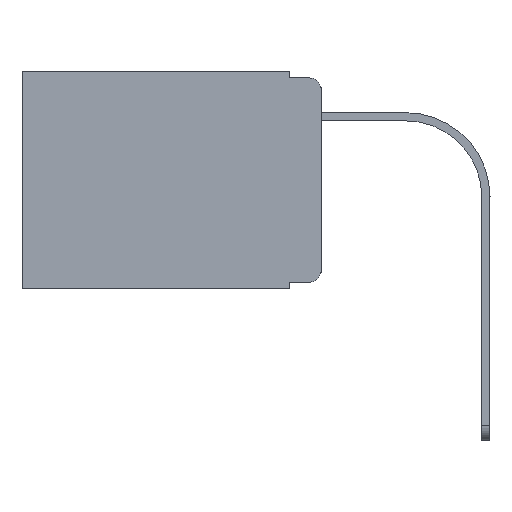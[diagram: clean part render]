
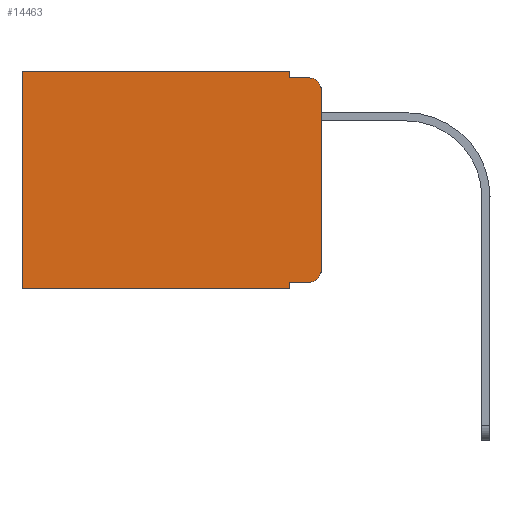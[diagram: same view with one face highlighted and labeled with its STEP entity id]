
A CAD part, left-side view. The second image highlights one B-rep face of the part: STEP entity #14463.
In plain terms, the highlighted planar face has unit normal (-1, 0, 0).
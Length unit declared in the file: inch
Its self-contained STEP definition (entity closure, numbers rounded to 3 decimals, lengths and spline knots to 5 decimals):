
#223 = CARTESIAN_POINT ( 'NONE',  ( 0.298, 0.051, -0.343 ) ) ;
#326 = EDGE_CURVE ( 'NONE', #18055, #405, #14141, .T. ) ;
#405 = VERTEX_POINT ( 'NONE', #223 ) ;
#505 = DIRECTION ( 'NONE',  ( 0., -1., 0. ) ) ;
#892 = DIRECTION ( 'NONE',  ( 0., 0., -1. ) ) ;
#959 = ORIENTED_EDGE ( 'NONE', *, *, #8449, .T. ) ;
#1194 = EDGE_CURVE ( 'NONE', #11760, #6548, #15734, .T. ) ;
#1338 = VERTEX_POINT ( 'NONE', #5907 ) ;
#1378 = DIRECTION ( 'NONE',  ( 0., 0., -1. ) ) ;
#1798 = FACE_OUTER_BOUND ( 'NONE', #3406, .T. ) ;
#2036 = VECTOR ( 'NONE', #18514, 39.37008 ) ;
#2287 = CARTESIAN_POINT ( 'NONE',  ( 0.298, 0., -0.343 ) ) ;
#2898 = DIRECTION ( 'NONE',  ( -1., 0., 0. ) ) ;
#3130 = DIRECTION ( 'NONE',  ( -1., 0., 0. ) ) ;
#3148 = VERTEX_POINT ( 'NONE', #5016 ) ;
#3279 = VECTOR ( 'NONE', #8430, 39.37008 ) ;
#3323 = CARTESIAN_POINT ( 'NONE',  ( 0.298, 0., 0. ) ) ;
#3406 = EDGE_LOOP ( 'NONE', ( #13383, #18698, #4146, #14200, #959, #3920, #7144, #18439, #6387, #9350 ) ) ;
#3530 = DIRECTION ( 'NONE',  ( 0., -1., 0. ) ) ;
#3554 = VECTOR ( 'NONE', #1378, 39.37008 ) ;
#3920 = ORIENTED_EDGE ( 'NONE', *, *, #1194, .T. ) ;
#3970 = VERTEX_POINT ( 'NONE', #10980 ) ;
#4146 = ORIENTED_EDGE ( 'NONE', *, *, #13550, .F. ) ;
#4601 = VECTOR ( 'NONE', #12641, 39.37008 ) ;
#4759 = VECTOR ( 'NONE', #505, 39.37008 ) ;
#4963 = LINE ( 'NONE', #7815, #9083 ) ;
#5016 = CARTESIAN_POINT ( 'NONE',  ( 0.298, 0., -0.03 ) ) ;
#5543 = LINE ( 'NONE', #2287, #2036 ) ;
#5906 = CARTESIAN_POINT ( 'NONE',  ( 0.298, 0.473, 0. ) ) ;
#5907 = CARTESIAN_POINT ( 'NONE',  ( 0.298, 0., -0.313 ) ) ;
#6193 = DIRECTION ( 'NONE',  ( 0., 0., -1. ) ) ;
#6314 = DIRECTION ( 'NONE',  ( 0., 1., 0. ) ) ;
#6387 = ORIENTED_EDGE ( 'NONE', *, *, #10122, .T. ) ;
#6539 = AXIS2_PLACEMENT_3D ( 'NONE', #17999, #3130, #7419 ) ;
#6548 = VERTEX_POINT ( 'NONE', #8036 ) ;
#6811 = CARTESIAN_POINT ( 'NONE',  ( 0.298, 0.051, 0. ) ) ;
#7144 = ORIENTED_EDGE ( 'NONE', *, *, #14064, .F. ) ;
#7419 = DIRECTION ( 'NONE',  ( 0., 0., -1. ) ) ;
#7556 = EDGE_CURVE ( 'NONE', #18207, #1338, #9958, .T. ) ;
#7567 = EDGE_CURVE ( 'NONE', #12636, #14679, #10074, .T. ) ;
#7608 = PLANE ( 'NONE',  #8438 ) ;
#7815 = CARTESIAN_POINT ( 'NONE',  ( 0.298, 0.051, -0.333 ) ) ;
#7850 = VECTOR ( 'NONE', #6314, 39.37008 ) ;
#7851 = LINE ( 'NONE', #11117, #18290 ) ;
#7915 = EDGE_CURVE ( 'NONE', #3148, #1338, #7851, .T. ) ;
#8036 = CARTESIAN_POINT ( 'NONE',  ( 0.298, 0.473, -0.343 ) ) ;
#8372 = CARTESIAN_POINT ( 'NONE',  ( 0.298, 0.051, -0.333 ) ) ;
#8430 = DIRECTION ( 'NONE',  ( 0., 0., -1. ) ) ;
#8438 = AXIS2_PLACEMENT_3D ( 'NONE', #3323, #18110, #6193 ) ;
#8449 = EDGE_CURVE ( 'NONE', #12636, #11760, #9181, .T. ) ;
#9083 = VECTOR ( 'NONE', #3530, 39.37008 ) ;
#9181 = LINE ( 'NONE', #17942, #7850 ) ;
#9350 = ORIENTED_EDGE ( 'NONE', *, *, #7556, .T. ) ;
#9958 = CIRCLE ( 'NONE', #18896, 0.02 ) ;
#10074 = LINE ( 'NONE', #18841, #3554 ) ;
#10122 = EDGE_CURVE ( 'NONE', #18055, #18207, #4963, .T. ) ;
#10980 = CARTESIAN_POINT ( 'NONE',  ( 0.298, 0.02, -0.01 ) ) ;
#11117 = CARTESIAN_POINT ( 'NONE',  ( 0.298, 0., 0. ) ) ;
#11236 = DIRECTION ( 'NONE',  ( 0., 0., -1. ) ) ;
#11442 = CARTESIAN_POINT ( 'NONE',  ( 0.298, 0.051, -0.01 ) ) ;
#11522 = CARTESIAN_POINT ( 'NONE',  ( 0.298, 0.02, -0.313 ) ) ;
#11734 = CARTESIAN_POINT ( 'NONE',  ( 0.298, 0.02, -0.333 ) ) ;
#11735 = CIRCLE ( 'NONE', #6539, 0.02 ) ;
#11760 = VERTEX_POINT ( 'NONE', #5906 ) ;
#11774 = EDGE_CURVE ( 'NONE', #3148, #3970, #11735, .T. ) ;
#12636 = VERTEX_POINT ( 'NONE', #16598 ) ;
#12641 = DIRECTION ( 'NONE',  ( 0., 0., -1. ) ) ;
#13383 = ORIENTED_EDGE ( 'NONE', *, *, #7915, .F. ) ;
#13550 = EDGE_CURVE ( 'NONE', #14679, #3970, #16524, .T. ) ;
#14064 = EDGE_CURVE ( 'NONE', #405, #6548, #5543, .T. ) ;
#14141 = LINE ( 'NONE', #6811, #3279 ) ;
#14200 = ORIENTED_EDGE ( 'NONE', *, *, #7567, .F. ) ;
#14463 = ADVANCED_FACE ( 'NONE', ( #1798 ), #7608, .F. ) ;
#14679 = VERTEX_POINT ( 'NONE', #11442 ) ;
#15734 = LINE ( 'NONE', #17172, #4601 ) ;
#16428 = CARTESIAN_POINT ( 'NONE',  ( 0.298, 0.051, -0.01 ) ) ;
#16524 = LINE ( 'NONE', #16428, #4759 ) ;
#16598 = CARTESIAN_POINT ( 'NONE',  ( 0.298, 0.051, 0. ) ) ;
#17172 = CARTESIAN_POINT ( 'NONE',  ( 0.298, 0.473, 0. ) ) ;
#17942 = CARTESIAN_POINT ( 'NONE',  ( 0.298, 0., 0. ) ) ;
#17999 = CARTESIAN_POINT ( 'NONE',  ( 0.298, 0.02, -0.03 ) ) ;
#18055 = VERTEX_POINT ( 'NONE', #8372 ) ;
#18110 = DIRECTION ( 'NONE',  ( 1., 0., 0. ) ) ;
#18207 = VERTEX_POINT ( 'NONE', #11734 ) ;
#18290 = VECTOR ( 'NONE', #892, 39.37008 ) ;
#18439 = ORIENTED_EDGE ( 'NONE', *, *, #326, .F. ) ;
#18514 = DIRECTION ( 'NONE',  ( 0., 1., 0. ) ) ;
#18698 = ORIENTED_EDGE ( 'NONE', *, *, #11774, .T. ) ;
#18841 = CARTESIAN_POINT ( 'NONE',  ( 0.298, 0.051, 0. ) ) ;
#18896 = AXIS2_PLACEMENT_3D ( 'NONE', #11522, #2898, #11236 ) ;
